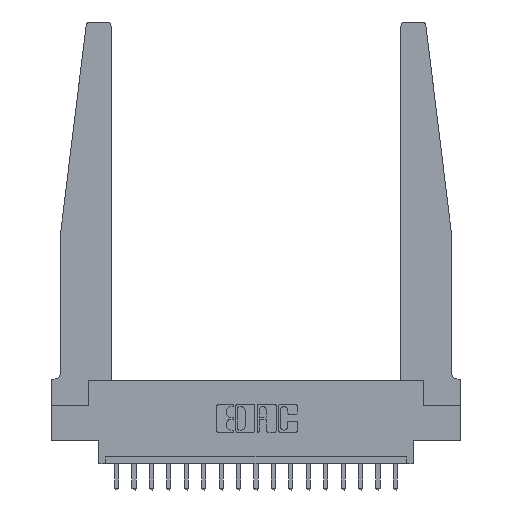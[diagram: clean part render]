
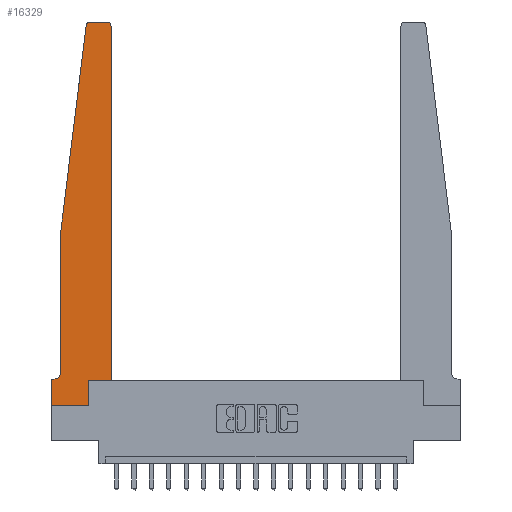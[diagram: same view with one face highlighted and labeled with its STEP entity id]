
A CAD part, top view. The second image highlights one B-rep face of the part: STEP entity #16329.
In plain terms, the highlighted planar face has unit normal (0, 0, 1).
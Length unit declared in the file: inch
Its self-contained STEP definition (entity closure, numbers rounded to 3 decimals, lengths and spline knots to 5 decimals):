
#101 = CARTESIAN_POINT ( 'NONE',  ( 0., 0.1875, 0.37 ) ) ;
#166 = VERTEX_POINT ( 'NONE', #13460 ) ;
#407 = CARTESIAN_POINT ( 'NONE',  ( 0.065, 0.1875, 0.37 ) ) ;
#603 = LINE ( 'NONE', #2268, #3584 ) ;
#744 = CARTESIAN_POINT ( 'NONE',  ( 0.065, 1.25, 0.37 ) ) ;
#1097 = ORIENTED_EDGE ( 'NONE', *, *, #17664, .T. ) ;
#1196 = ORIENTED_EDGE ( 'NONE', *, *, #4283, .T. ) ;
#1291 = DIRECTION ( 'NONE',  ( 0., -1., 0. ) ) ;
#1383 = CARTESIAN_POINT ( 'NONE',  ( 0., 0., 0.37 ) ) ;
#1410 = VECTOR ( 'NONE', #7046, 39.37008 ) ;
#1510 = VERTEX_POINT ( 'NONE', #8525 ) ;
#1628 = VERTEX_POINT ( 'NONE', #4410 ) ;
#1674 = DIRECTION ( 'NONE',  ( 0., 0., 1. ) ) ;
#1679 = CARTESIAN_POINT ( 'NONE',  ( 0.24675, 2.72367, 0.37 ) ) ;
#2177 = CARTESIAN_POINT ( 'NONE',  ( 0.065, 0.2375, 0.37 ) ) ;
#2268 = CARTESIAN_POINT ( 'NONE',  ( 0.065, 1.25, 0.37 ) ) ;
#2321 = VERTEX_POINT ( 'NONE', #8774 ) ;
#2338 = CARTESIAN_POINT ( 'NONE',  ( 0.25, 2.75, 0.37 ) ) ;
#2787 = ORIENTED_EDGE ( 'NONE', *, *, #6036, .T. ) ;
#3156 = LINE ( 'NONE', #407, #12962 ) ;
#3199 = CARTESIAN_POINT ( 'NONE',  ( 0.425, 0.18, 0.37 ) ) ;
#3361 = DIRECTION ( 'NONE',  ( 0., 1., 0. ) ) ;
#3560 = CARTESIAN_POINT ( 'NONE',  ( 0.425, 0.18, 0.37 ) ) ;
#3584 = VECTOR ( 'NONE', #3825, 39.37008 ) ;
#3699 = EDGE_CURVE ( 'NONE', #7182, #4922, #18239, .T. ) ;
#3825 = DIRECTION ( 'NONE',  ( -0.122, -0.992, 0. ) ) ;
#4233 = CIRCLE ( 'NONE', #18343, 0.03 ) ;
#4283 = EDGE_CURVE ( 'NONE', #9436, #1628, #603, .T. ) ;
#4322 = VERTEX_POINT ( 'NONE', #18930 ) ;
#4370 = CARTESIAN_POINT ( 'NONE',  ( 0.425, 0.18, 0.37 ) ) ;
#4410 = CARTESIAN_POINT ( 'NONE',  ( 0.065, 1.25, 0.37 ) ) ;
#4554 = EDGE_CURVE ( 'NONE', #2321, #9436, #4233, .T. ) ;
#4812 = DIRECTION ( 'NONE',  ( -1., 0., 0. ) ) ;
#4922 = VERTEX_POINT ( 'NONE', #12472 ) ;
#5340 = VERTEX_POINT ( 'NONE', #15787 ) ;
#5592 = EDGE_CURVE ( 'NONE', #8256, #4322, #17023, .T. ) ;
#5758 = CARTESIAN_POINT ( 'NONE',  ( 0., 0., 0.37 ) ) ;
#5952 = DIRECTION ( 'NONE',  ( 1., 0., 0. ) ) ;
#6036 = EDGE_CURVE ( 'NONE', #5340, #15456, #7788, .T. ) ;
#6127 = CARTESIAN_POINT ( 'NONE',  ( 0.015, 0.2375, 0.37 ) ) ;
#6271 = VECTOR ( 'NONE', #3361, 39.37008 ) ;
#7046 = DIRECTION ( 'NONE',  ( -1., 0., 0. ) ) ;
#7182 = VERTEX_POINT ( 'NONE', #2177 ) ;
#7297 = EDGE_LOOP ( 'NONE', ( #8326, #18257, #1196, #7494, #16569, #1097, #18693, #18180, #2787, #16864, #15560, #15613 ) ) ;
#7494 = ORIENTED_EDGE ( 'NONE', *, *, #15356, .T. ) ;
#7620 = AXIS2_PLACEMENT_3D ( 'NONE', #101, #9109, #16583 ) ;
#7641 = VERTEX_POINT ( 'NONE', #17174 ) ;
#7788 = LINE ( 'NONE', #18273, #6271 ) ;
#8256 = VERTEX_POINT ( 'NONE', #4370 ) ;
#8326 = ORIENTED_EDGE ( 'NONE', *, *, #18542, .T. ) ;
#8525 = CARTESIAN_POINT ( 'NONE',  ( 0., 0., 0.37 ) ) ;
#8774 = CARTESIAN_POINT ( 'NONE',  ( 0.27653, 2.75, 0.37 ) ) ;
#9109 = DIRECTION ( 'NONE',  ( 0., 0., 1. ) ) ;
#9146 = VECTOR ( 'NONE', #5952, 39.37008 ) ;
#9358 = EDGE_CURVE ( 'NONE', #166, #1510, #10013, .T. ) ;
#9406 = VECTOR ( 'NONE', #1291, 39.37008 ) ;
#9436 = VERTEX_POINT ( 'NONE', #1679 ) ;
#9629 = CARTESIAN_POINT ( 'NONE',  ( 0.395, 2.72, 0.37 ) ) ;
#9730 = CIRCLE ( 'NONE', #10994, 0.03 ) ;
#10013 = LINE ( 'NONE', #1383, #9406 ) ;
#10174 = VECTOR ( 'NONE', #12141, 39.37008 ) ;
#10178 = LINE ( 'NONE', #5758, #9146 ) ;
#10994 = AXIS2_PLACEMENT_3D ( 'NONE', #9629, #12686, #15633 ) ;
#11443 = DIRECTION ( 'NONE',  ( 0., -1., 0. ) ) ;
#11827 = CARTESIAN_POINT ( 'NONE',  ( 0.2605, 0.18, 0.37 ) ) ;
#12122 = DIRECTION ( 'NONE',  ( 0., 0., -1. ) ) ;
#12141 = DIRECTION ( 'NONE',  ( 1., 0., 0. ) ) ;
#12309 = EDGE_CURVE ( 'NONE', #4322, #7641, #9730, .T. ) ;
#12472 = CARTESIAN_POINT ( 'NONE',  ( 0.015, 0.1875, 0.37 ) ) ;
#12686 = DIRECTION ( 'NONE',  ( 0., 0., 1. ) ) ;
#12962 = VECTOR ( 'NONE', #4812, 39.37008 ) ;
#13460 = CARTESIAN_POINT ( 'NONE',  ( 0., 0.1875, 0.37 ) ) ;
#13540 = CARTESIAN_POINT ( 'NONE',  ( 0.27653, 2.72, 0.37 ) ) ;
#13582 = VECTOR ( 'NONE', #11443, 39.37008 ) ;
#13842 = EDGE_CURVE ( 'NONE', #1510, #5340, #10178, .T. ) ;
#14610 = LINE ( 'NONE', #2338, #1410 ) ;
#14890 = LINE ( 'NONE', #3199, #10174 ) ;
#15214 = FACE_OUTER_BOUND ( 'NONE', #7297, .T. ) ;
#15356 = EDGE_CURVE ( 'NONE', #1628, #7182, #15666, .T. ) ;
#15456 = VERTEX_POINT ( 'NONE', #11827 ) ;
#15560 = ORIENTED_EDGE ( 'NONE', *, *, #5592, .T. ) ;
#15613 = ORIENTED_EDGE ( 'NONE', *, *, #12309, .T. ) ;
#15633 = DIRECTION ( 'NONE',  ( 1., 0., 0. ) ) ;
#15666 = LINE ( 'NONE', #744, #13582 ) ;
#15787 = CARTESIAN_POINT ( 'NONE',  ( 0.2605, 0., 0.37 ) ) ;
#16329 = ADVANCED_FACE ( 'NONE', ( #15214 ), #16683, .T. ) ;
#16569 = ORIENTED_EDGE ( 'NONE', *, *, #3699, .T. ) ;
#16576 = VECTOR ( 'NONE', #16838, 39.37008 ) ;
#16583 = DIRECTION ( 'NONE',  ( 1., 0., 0. ) ) ;
#16674 = AXIS2_PLACEMENT_3D ( 'NONE', #6127, #12122, #18105 ) ;
#16683 = PLANE ( 'NONE',  #7620 ) ;
#16838 = DIRECTION ( 'NONE',  ( 0., 1., 0. ) ) ;
#16864 = ORIENTED_EDGE ( 'NONE', *, *, #18660, .T. ) ;
#17023 = LINE ( 'NONE', #3560, #16576 ) ;
#17174 = CARTESIAN_POINT ( 'NONE',  ( 0.395, 2.75, 0.37 ) ) ;
#17664 = EDGE_CURVE ( 'NONE', #4922, #166, #3156, .T. ) ;
#18061 = DIRECTION ( 'NONE',  ( 1., 0., 0. ) ) ;
#18105 = DIRECTION ( 'NONE',  ( -1., 0., 0. ) ) ;
#18180 = ORIENTED_EDGE ( 'NONE', *, *, #13842, .T. ) ;
#18239 = CIRCLE ( 'NONE', #16674, 0.05 ) ;
#18257 = ORIENTED_EDGE ( 'NONE', *, *, #4554, .T. ) ;
#18273 = CARTESIAN_POINT ( 'NONE',  ( 0.2605, 0.18, 0.37 ) ) ;
#18343 = AXIS2_PLACEMENT_3D ( 'NONE', #13540, #1674, #18061 ) ;
#18542 = EDGE_CURVE ( 'NONE', #7641, #2321, #14610, .T. ) ;
#18660 = EDGE_CURVE ( 'NONE', #15456, #8256, #14890, .T. ) ;
#18693 = ORIENTED_EDGE ( 'NONE', *, *, #9358, .T. ) ;
#18930 = CARTESIAN_POINT ( 'NONE',  ( 0.425, 2.72, 0.37 ) ) ;
